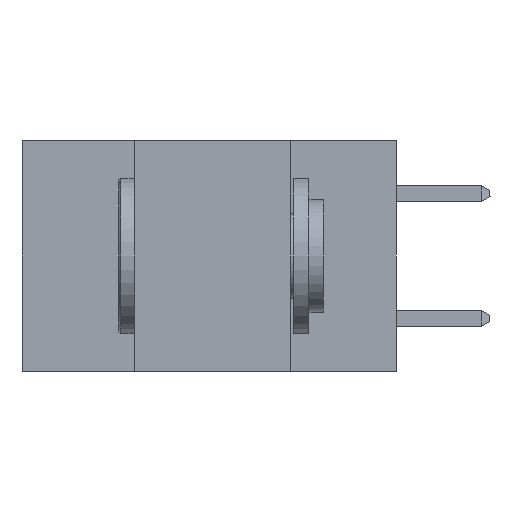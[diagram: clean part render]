
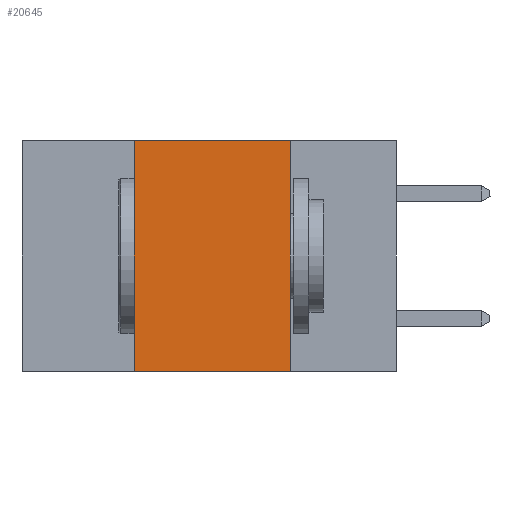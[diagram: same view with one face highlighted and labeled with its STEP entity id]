
A CAD part, left-side view. The second image highlights one B-rep face of the part: STEP entity #20645.
In plain terms, the highlighted planar face has unit normal (-1, 0, 0).
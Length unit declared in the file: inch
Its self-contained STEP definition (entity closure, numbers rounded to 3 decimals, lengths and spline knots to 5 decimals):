
#439 = ORIENTED_EDGE ( 'NONE', *, *, #2216, .F. ) ;
#1617 = DIRECTION ( 'NONE',  ( 0., -1., 0. ) ) ;
#2216 = EDGE_CURVE ( 'NONE', #16244, #6885, #15800, .T. ) ;
#6885 = VERTEX_POINT ( 'NONE', #22039 ) ;
#7317 = DIRECTION ( 'NONE',  ( 0., 0., -1. ) ) ;
#7495 = CARTESIAN_POINT ( 'NONE',  ( 0., 0.42, -0.37 ) ) ;
#7718 = AXIS2_PLACEMENT_3D ( 'NONE', #10991, #13077, #12897 ) ;
#9229 = VECTOR ( 'NONE', #1617, 39.37008 ) ;
#10880 = LINE ( 'NONE', #16712, #9229 ) ;
#10991 = CARTESIAN_POINT ( 'NONE',  ( 0., 0.6, 0. ) ) ;
#12608 = DIRECTION ( 'NONE',  ( 0., 0., 1. ) ) ;
#12897 = DIRECTION ( 'NONE',  ( 0., 0., -1. ) ) ;
#13077 = DIRECTION ( 'NONE',  ( 1., 0., 0. ) ) ;
#14456 = VECTOR ( 'NONE', #12608, 39.37008 ) ;
#14674 = ORIENTED_EDGE ( 'NONE', *, *, #24186, .T. ) ;
#15800 = LINE ( 'NONE', #19106, #14456 ) ;
#16244 = VERTEX_POINT ( 'NONE', #7495 ) ;
#16712 = CARTESIAN_POINT ( 'NONE',  ( 0., 0.6, -0.37 ) ) ;
#16960 = VERTEX_POINT ( 'NONE', #17369 ) ;
#17369 = CARTESIAN_POINT ( 'NONE',  ( 0., 0.17, -0.37 ) ) ;
#17413 = ORIENTED_EDGE ( 'NONE', *, *, #23221, .F. ) ;
#17448 = LINE ( 'NONE', #24542, #22883 ) ;
#17690 = LINE ( 'NONE', #28016, #26152 ) ;
#18148 = CARTESIAN_POINT ( 'NONE',  ( 0., 0.17, 0. ) ) ;
#19106 = CARTESIAN_POINT ( 'NONE',  ( 0., 0.42, 0. ) ) ;
#20049 = EDGE_LOOP ( 'NONE', ( #17413, #23820, #439, #14674 ) ) ;
#20645 = ADVANCED_FACE ( 'NONE', ( #20991 ), #21830, .F. ) ;
#20991 = FACE_OUTER_BOUND ( 'NONE', #20049, .T. ) ;
#21830 = PLANE ( 'NONE',  #7718 ) ;
#22039 = CARTESIAN_POINT ( 'NONE',  ( 0., 0.42, 0. ) ) ;
#22883 = VECTOR ( 'NONE', #7317, 39.37008 ) ;
#23221 = EDGE_CURVE ( 'NONE', #26872, #16960, #17448, .T. ) ;
#23335 = DIRECTION ( 'NONE',  ( 0., -1., 0. ) ) ;
#23820 = ORIENTED_EDGE ( 'NONE', *, *, #26358, .F. ) ;
#24186 = EDGE_CURVE ( 'NONE', #16244, #16960, #10880, .T. ) ;
#24542 = CARTESIAN_POINT ( 'NONE',  ( 0., 0.17, 0. ) ) ;
#26152 = VECTOR ( 'NONE', #23335, 39.37008 ) ;
#26358 = EDGE_CURVE ( 'NONE', #6885, #26872, #17690, .T. ) ;
#26872 = VERTEX_POINT ( 'NONE', #18148 ) ;
#28016 = CARTESIAN_POINT ( 'NONE',  ( 0., 0.6, 0. ) ) ;
